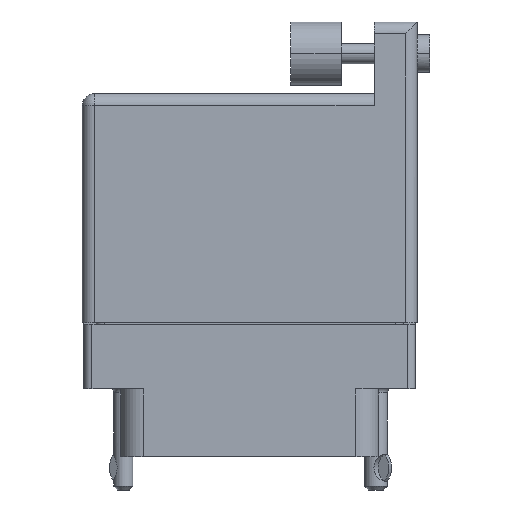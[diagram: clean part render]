
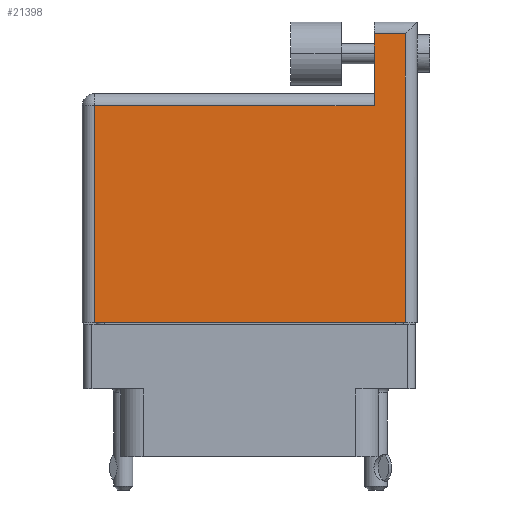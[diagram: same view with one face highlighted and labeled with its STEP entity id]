
A CAD part, front view. The second image highlights one B-rep face of the part: STEP entity #21398.
In plain terms, the highlighted face is planar.
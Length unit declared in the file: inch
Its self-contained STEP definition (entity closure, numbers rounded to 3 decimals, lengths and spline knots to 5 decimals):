
#97 = LINE ( 'NONE', #36013, #30430 ) ;
#2136 = DIRECTION ( 'NONE',  ( 0., 0., -1. ) ) ;
#2232 = EDGE_LOOP ( 'NONE', ( #33494, #3737, #8335, #10136, #11136, #13696 ) ) ;
#2966 = CARTESIAN_POINT ( 'NONE',  ( 0.4925, 1.043, 0.3575 ) ) ;
#3737 = ORIENTED_EDGE ( 'NONE', *, *, #5111, .T. ) ;
#4684 = DIRECTION ( 'NONE',  ( 0., -1., 0. ) ) ;
#5111 = EDGE_CURVE ( 'NONE', #37731, #34577, #18551, .T. ) ;
#5325 = LINE ( 'NONE', #25971, #17371 ) ;
#5568 = EDGE_CURVE ( 'NONE', #6998, #39519, #35337, .T. ) ;
#6194 = LINE ( 'NONE', #18281, #25012 ) ;
#6998 = VERTEX_POINT ( 'NONE', #36552 ) ;
#7883 = EDGE_CURVE ( 'NONE', #34841, #6998, #5325, .T. ) ;
#8335 = ORIENTED_EDGE ( 'NONE', *, *, #24784, .T. ) ;
#8587 = CARTESIAN_POINT ( 'NONE',  ( -0.6625, 0.806, 0.3575 ) ) ;
#9783 = CARTESIAN_POINT ( 'NONE',  ( -0.6155, -0.1, 0.3575 ) ) ;
#10136 = ORIENTED_EDGE ( 'NONE', *, *, #7883, .T. ) ;
#10347 = CARTESIAN_POINT ( 'NONE',  ( 0.6155, 1.09, 0.3575 ) ) ;
#10568 = CARTESIAN_POINT ( 'NONE',  ( -0.6155, -0.1, 0.3575 ) ) ;
#10786 = VECTOR ( 'NONE', #10955, 39.37008 ) ;
#10955 = DIRECTION ( 'NONE',  ( -1., 0., 0. ) ) ;
#11074 = CARTESIAN_POINT ( 'NONE',  ( -0.6625, 0.759, 0.3575 ) ) ;
#11136 = ORIENTED_EDGE ( 'NONE', *, *, #5568, .T. ) ;
#11696 = PLANE ( 'NONE',  #13736 ) ;
#13696 = ORIENTED_EDGE ( 'NONE', *, *, #21647, .T. ) ;
#13736 = AXIS2_PLACEMENT_3D ( 'NONE', #8587, #2136, #30159 ) ;
#13746 = EDGE_CURVE ( 'NONE', #35623, #37731, #97, .T. ) ;
#14202 = VECTOR ( 'NONE', #16714, 39.37008 ) ;
#16520 = VECTOR ( 'NONE', #22208, 39.37008 ) ;
#16714 = DIRECTION ( 'NONE',  ( 0., 1., 0. ) ) ;
#17371 = VECTOR ( 'NONE', #4684, 39.37008 ) ;
#18281 = CARTESIAN_POINT ( 'NONE',  ( 0.4925, 1.043, 0.3575 ) ) ;
#18551 = LINE ( 'NONE', #10347, #14202 ) ;
#21398 = ADVANCED_FACE ( 'NONE', ( #37223 ), #11696, .F. ) ;
#21647 = EDGE_CURVE ( 'NONE', #39519, #35623, #35233, .T. ) ;
#22208 = DIRECTION ( 'NONE',  ( 0., -1., 0. ) ) ;
#24784 = EDGE_CURVE ( 'NONE', #34577, #34841, #6194, .T. ) ;
#25012 = VECTOR ( 'NONE', #36941, 39.37008 ) ;
#25971 = CARTESIAN_POINT ( 'NONE',  ( 0.4925, 1.09, 0.3575 ) ) ;
#29068 = CARTESIAN_POINT ( 'NONE',  ( -0.6155, 0.759, 0.3575 ) ) ;
#30159 = DIRECTION ( 'NONE',  ( -1., 0., 0. ) ) ;
#30430 = VECTOR ( 'NONE', #39142, 39.37008 ) ;
#33494 = ORIENTED_EDGE ( 'NONE', *, *, #13746, .T. ) ;
#34577 = VERTEX_POINT ( 'NONE', #39799 ) ;
#34841 = VERTEX_POINT ( 'NONE', #2966 ) ;
#35233 = LINE ( 'NONE', #9783, #16520 ) ;
#35337 = LINE ( 'NONE', #11074, #10786 ) ;
#35623 = VERTEX_POINT ( 'NONE', #10568 ) ;
#36013 = CARTESIAN_POINT ( 'NONE',  ( -0.6625, -0.1, 0.3575 ) ) ;
#36552 = CARTESIAN_POINT ( 'NONE',  ( 0.4925, 0.759, 0.3575 ) ) ;
#36941 = DIRECTION ( 'NONE',  ( -1., 0., 0. ) ) ;
#37223 = FACE_OUTER_BOUND ( 'NONE', #2232, .T. ) ;
#37731 = VERTEX_POINT ( 'NONE', #38413 ) ;
#38413 = CARTESIAN_POINT ( 'NONE',  ( 0.6155, -0.1, 0.3575 ) ) ;
#39142 = DIRECTION ( 'NONE',  ( 1., 0., 0. ) ) ;
#39519 = VERTEX_POINT ( 'NONE', #29068 ) ;
#39799 = CARTESIAN_POINT ( 'NONE',  ( 0.6155, 1.043, 0.3575 ) ) ;
